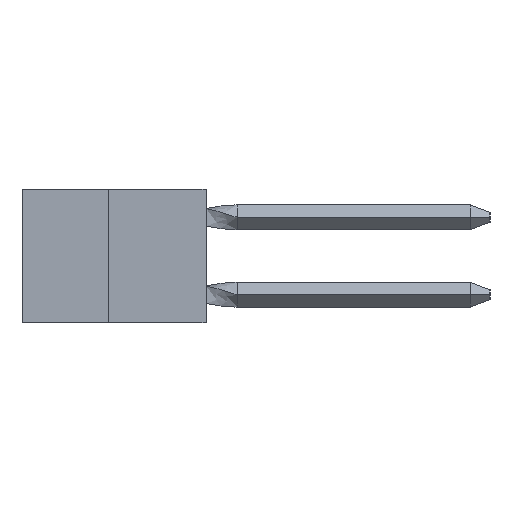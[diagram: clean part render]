
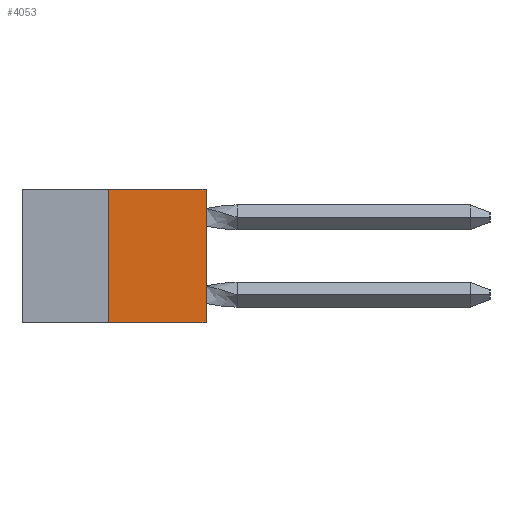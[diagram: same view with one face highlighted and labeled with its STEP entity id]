
A CAD part, left-side view. The second image highlights one B-rep face of the part: STEP entity #4053.
In plain terms, the highlighted planar face has unit normal (-1, 0, 0).
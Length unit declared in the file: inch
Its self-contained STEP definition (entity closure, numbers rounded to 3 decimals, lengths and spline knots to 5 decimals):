
#741 = EDGE_CURVE ( 'NONE', #19551, #5306, #2342, .T. ) ;
#1171 = LINE ( 'NONE', #13305, #22475 ) ;
#1325 = DIRECTION ( 'NONE',  ( 0., 0., 1. ) ) ;
#1709 = DIRECTION ( 'NONE',  ( 0., 0., -1. ) ) ;
#1710 = ORIENTED_EDGE ( 'NONE', *, *, #741, .F. ) ;
#2342 = LINE ( 'NONE', #11957, #13695 ) ;
#2787 = CARTESIAN_POINT ( 'NONE',  ( 0., 0., 0. ) ) ;
#3295 = CARTESIAN_POINT ( 'NONE',  ( 0., 0., 0. ) ) ;
#3787 = AXIS2_PLACEMENT_3D ( 'NONE', #7125, #19537, #1709 ) ;
#3964 = VERTEX_POINT ( 'NONE', #3295 ) ;
#4053 = ADVANCED_FACE ( 'NONE', ( #11632 ), #5380, .F. ) ;
#5188 = ORIENTED_EDGE ( 'NONE', *, *, #8689, .T. ) ;
#5306 = VERTEX_POINT ( 'NONE', #17217 ) ;
#5380 = PLANE ( 'NONE',  #3787 ) ;
#5806 = CARTESIAN_POINT ( 'NONE',  ( 0., 0.25, -0.343 ) ) ;
#5928 = VECTOR ( 'NONE', #15750, 39.37008 ) ;
#5954 = LINE ( 'NONE', #14274, #5928 ) ;
#7108 = ORIENTED_EDGE ( 'NONE', *, *, #21370, .F. ) ;
#7125 = CARTESIAN_POINT ( 'NONE',  ( 0., 0.473, 0. ) ) ;
#8689 = EDGE_CURVE ( 'NONE', #19551, #8996, #5954, .T. ) ;
#8996 = VERTEX_POINT ( 'NONE', #20955 ) ;
#9415 = EDGE_CURVE ( 'NONE', #8996, #3964, #18650, .T. ) ;
#9759 = VECTOR ( 'NONE', #11770, 39.37008 ) ;
#11632 = FACE_OUTER_BOUND ( 'NONE', #14079, .T. ) ;
#11770 = DIRECTION ( 'NONE',  ( 0., 0., 1. ) ) ;
#11957 = CARTESIAN_POINT ( 'NONE',  ( 0., 0.25, 0. ) ) ;
#12830 = ORIENTED_EDGE ( 'NONE', *, *, #9415, .T. ) ;
#13305 = CARTESIAN_POINT ( 'NONE',  ( 0., 0.473, 0. ) ) ;
#13695 = VECTOR ( 'NONE', #1325, 39.37008 ) ;
#14079 = EDGE_LOOP ( 'NONE', ( #7108, #1710, #5188, #12830 ) ) ;
#14274 = CARTESIAN_POINT ( 'NONE',  ( 0., 0.473, -0.343 ) ) ;
#15091 = DIRECTION ( 'NONE',  ( 0., -1., 0. ) ) ;
#15750 = DIRECTION ( 'NONE',  ( 0., -1., 0. ) ) ;
#17217 = CARTESIAN_POINT ( 'NONE',  ( 0., 0.25, 0. ) ) ;
#18650 = LINE ( 'NONE', #2787, #9759 ) ;
#19537 = DIRECTION ( 'NONE',  ( 1., 0., 0. ) ) ;
#19551 = VERTEX_POINT ( 'NONE', #5806 ) ;
#20955 = CARTESIAN_POINT ( 'NONE',  ( 0., 0., -0.343 ) ) ;
#21370 = EDGE_CURVE ( 'NONE', #5306, #3964, #1171, .T. ) ;
#22475 = VECTOR ( 'NONE', #15091, 39.37008 ) ;
